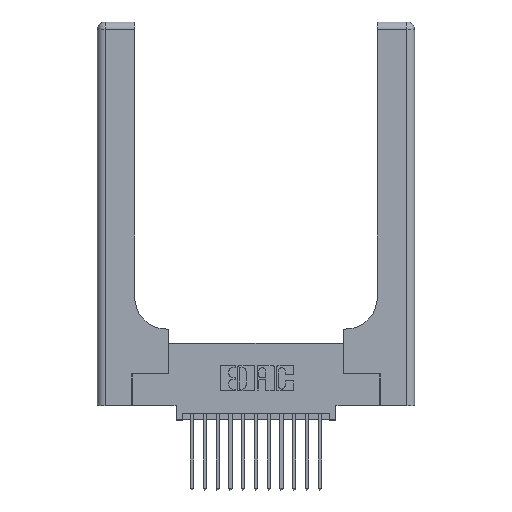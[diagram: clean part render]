
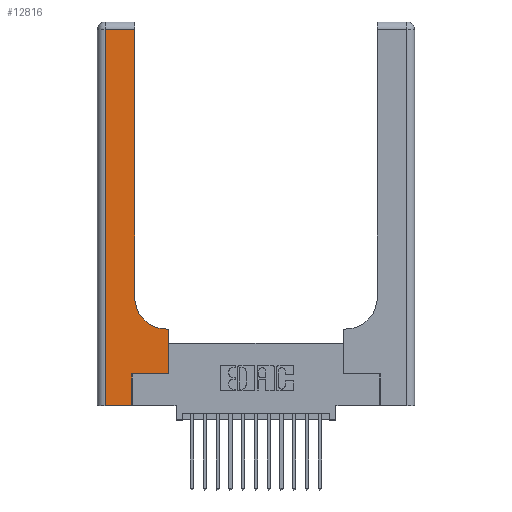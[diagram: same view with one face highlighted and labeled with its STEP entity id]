
A CAD part, top view. The second image highlights one B-rep face of the part: STEP entity #12816.
In plain terms, the highlighted planar face has unit normal (0, 0, 1).
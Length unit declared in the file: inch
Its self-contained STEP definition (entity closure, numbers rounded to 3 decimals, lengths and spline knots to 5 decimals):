
#737 = DIRECTION ( 'NONE',  ( 0., 0., -1. ) ) ;
#1330 = DIRECTION ( 'NONE',  ( 0., 0., -1. ) ) ;
#1965 = EDGE_CURVE ( 'NONE', #10799, #6505, #4202, .T. ) ;
#2408 = CARTESIAN_POINT ( 'NONE',  ( 0.06, 3., 0.37 ) ) ;
#2530 = CARTESIAN_POINT ( 'NONE',  ( 0.269, 0., 0.37 ) ) ;
#2596 = DIRECTION ( 'NONE',  ( -1., 0., 0. ) ) ;
#2600 = EDGE_CURVE ( 'NONE', #14567, #14166, #13449, .T. ) ;
#2721 = DIRECTION ( 'NONE',  ( -1., 0., 0. ) ) ;
#3223 = VERTEX_POINT ( 'NONE', #17330 ) ;
#3565 = LINE ( 'NONE', #4645, #10935 ) ;
#3674 = ORIENTED_EDGE ( 'NONE', *, *, #1965, .T. ) ;
#3700 = CARTESIAN_POINT ( 'NONE',  ( 0.5585, 0.25, 0.37 ) ) ;
#3914 = EDGE_CURVE ( 'NONE', #4624, #7304, #4469, .T. ) ;
#4045 = CARTESIAN_POINT ( 'NONE',  ( 0.2915, 0.6, 0.37 ) ) ;
#4197 = EDGE_CURVE ( 'NONE', #6505, #14567, #13845, .T. ) ;
#4202 = LINE ( 'NONE', #4045, #8528 ) ;
#4469 = LINE ( 'NONE', #2408, #10334 ) ;
#4624 = VERTEX_POINT ( 'NONE', #14397 ) ;
#4645 = CARTESIAN_POINT ( 'NONE',  ( 0.269, 0.25, 0.37 ) ) ;
#4772 = ORIENTED_EDGE ( 'NONE', *, *, #16612, .T. ) ;
#4837 = PLANE ( 'NONE',  #5106 ) ;
#5106 = AXIS2_PLACEMENT_3D ( 'NONE', #14612, #737, #6280 ) ;
#5211 = CARTESIAN_POINT ( 'NONE',  ( 0.2915, 2.94, 0.37 ) ) ;
#5294 = LINE ( 'NONE', #2530, #8544 ) ;
#5308 = EDGE_CURVE ( 'NONE', #7986, #10799, #10511, .T. ) ;
#5584 = CARTESIAN_POINT ( 'NONE',  ( 0.2915, 3., 0.37 ) ) ;
#5834 = ORIENTED_EDGE ( 'NONE', *, *, #7804, .T. ) ;
#5960 = CARTESIAN_POINT ( 'NONE',  ( 0., 0., 0.37 ) ) ;
#6280 = DIRECTION ( 'NONE',  ( -1., 0., 0. ) ) ;
#6505 = VERTEX_POINT ( 'NONE', #10919 ) ;
#7304 = VERTEX_POINT ( 'NONE', #14480 ) ;
#7443 = VECTOR ( 'NONE', #10669, 39.37008 ) ;
#7573 = ORIENTED_EDGE ( 'NONE', *, *, #3914, .T. ) ;
#7804 = EDGE_CURVE ( 'NONE', #7304, #3223, #13501, .T. ) ;
#7856 = DIRECTION ( 'NONE',  ( 0., -1., 0. ) ) ;
#7922 = CARTESIAN_POINT ( 'NONE',  ( 0.5585, 0.6, 0.37 ) ) ;
#7986 = VERTEX_POINT ( 'NONE', #15962 ) ;
#8363 = ORIENTED_EDGE ( 'NONE', *, *, #4197, .T. ) ;
#8525 = CARTESIAN_POINT ( 'NONE',  ( 0.2915, 0.85, 0.37 ) ) ;
#8528 = VECTOR ( 'NONE', #2596, 39.37008 ) ;
#8544 = VECTOR ( 'NONE', #15100, 39.37008 ) ;
#9115 = EDGE_CURVE ( 'NONE', #14374, #7986, #3565, .T. ) ;
#9418 = EDGE_CURVE ( 'NONE', #3223, #14374, #5294, .T. ) ;
#9827 = ORIENTED_EDGE ( 'NONE', *, *, #9115, .T. ) ;
#9870 = CARTESIAN_POINT ( 'NONE',  ( 0.269, 0.25, 0.37 ) ) ;
#10334 = VECTOR ( 'NONE', #7856, 39.37008 ) ;
#10511 = LINE ( 'NONE', #3700, #7443 ) ;
#10669 = DIRECTION ( 'NONE',  ( 0., 1., 0. ) ) ;
#10799 = VERTEX_POINT ( 'NONE', #7922 ) ;
#10843 = ORIENTED_EDGE ( 'NONE', *, *, #5308, .T. ) ;
#10919 = CARTESIAN_POINT ( 'NONE',  ( 0.5415, 0.6, 0.37 ) ) ;
#10935 = VECTOR ( 'NONE', #14552, 39.37008 ) ;
#12816 = ADVANCED_FACE ( 'NONE', ( #14389 ), #4837, .F. ) ;
#12949 = LINE ( 'NONE', #17894, #15370 ) ;
#13449 = LINE ( 'NONE', #5584, #14090 ) ;
#13501 = LINE ( 'NONE', #5960, #16582 ) ;
#13845 = CIRCLE ( 'NONE', #18069, 0.25 ) ;
#14090 = VECTOR ( 'NONE', #18096, 39.37008 ) ;
#14166 = VERTEX_POINT ( 'NONE', #5211 ) ;
#14374 = VERTEX_POINT ( 'NONE', #9870 ) ;
#14389 = FACE_OUTER_BOUND ( 'NONE', #16390, .T. ) ;
#14397 = CARTESIAN_POINT ( 'NONE',  ( 0.06, 2.94, 0.37 ) ) ;
#14480 = CARTESIAN_POINT ( 'NONE',  ( 0.06, 0., 0.37 ) ) ;
#14552 = DIRECTION ( 'NONE',  ( 1., 0., 0. ) ) ;
#14567 = VERTEX_POINT ( 'NONE', #8525 ) ;
#14612 = CARTESIAN_POINT ( 'NONE',  ( 0., 3., 0.37 ) ) ;
#15100 = DIRECTION ( 'NONE',  ( 0., 1., 0. ) ) ;
#15370 = VECTOR ( 'NONE', #2721, 39.37008 ) ;
#15962 = CARTESIAN_POINT ( 'NONE',  ( 0.5585, 0.25, 0.37 ) ) ;
#16390 = EDGE_LOOP ( 'NONE', ( #16946, #4772, #7573, #5834, #18013, #9827, #10843, #3674, #8363 ) ) ;
#16582 = VECTOR ( 'NONE', #17125, 39.37008 ) ;
#16612 = EDGE_CURVE ( 'NONE', #14166, #4624, #12949, .T. ) ;
#16925 = CARTESIAN_POINT ( 'NONE',  ( 0.5415, 0.85, 0.37 ) ) ;
#16946 = ORIENTED_EDGE ( 'NONE', *, *, #2600, .T. ) ;
#17125 = DIRECTION ( 'NONE',  ( 1., 0., 0. ) ) ;
#17330 = CARTESIAN_POINT ( 'NONE',  ( 0.269, 0., 0.37 ) ) ;
#17894 = CARTESIAN_POINT ( 'NONE',  ( 0., 2.94, 0.37 ) ) ;
#18013 = ORIENTED_EDGE ( 'NONE', *, *, #9418, .T. ) ;
#18069 = AXIS2_PLACEMENT_3D ( 'NONE', #16925, #1330, #18158 ) ;
#18096 = DIRECTION ( 'NONE',  ( 0., 1., 0. ) ) ;
#18158 = DIRECTION ( 'NONE',  ( 1., 0., 0. ) ) ;
